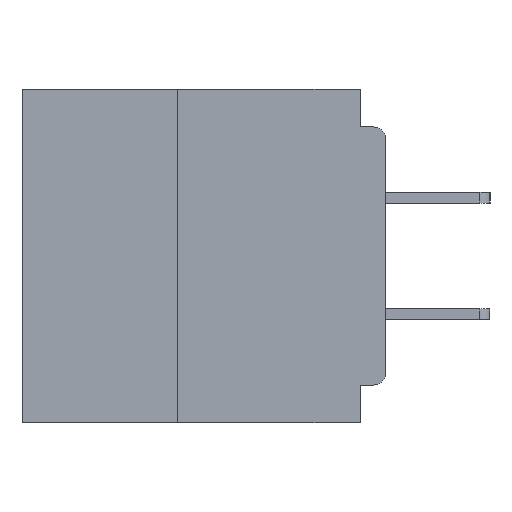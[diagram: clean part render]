
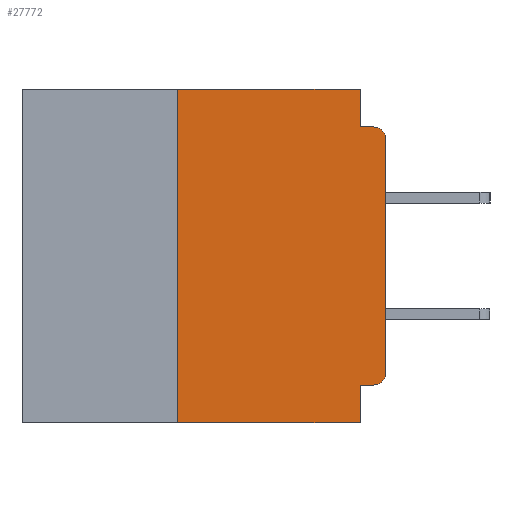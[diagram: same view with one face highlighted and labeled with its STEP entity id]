
A CAD part, left-side view. The second image highlights one B-rep face of the part: STEP entity #27772.
In plain terms, the highlighted planar face has unit normal (-1, 0, 0).
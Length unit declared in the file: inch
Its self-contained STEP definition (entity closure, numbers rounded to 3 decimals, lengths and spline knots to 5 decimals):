
#94 = VECTOR ( 'NONE', #56220, 39.37008 ) ;
#1191 = EDGE_CURVE ( 'NONE', #36905, #11573, #17959, .T. ) ;
#1698 = CARTESIAN_POINT ( 'NONE',  ( 0., 0.437, 0. ) ) ;
#2659 = VECTOR ( 'NONE', #55252, 39.37008 ) ;
#3322 = DIRECTION ( 'NONE',  ( 0., -1., 0. ) ) ;
#4088 = LINE ( 'NONE', #19762, #2659 ) ;
#4340 = CARTESIAN_POINT ( 'NONE',  ( 0., 0.015, -0.34 ) ) ;
#6059 = DIRECTION ( 'NONE',  ( 0., -1., 0. ) ) ;
#6978 = ORIENTED_EDGE ( 'NONE', *, *, #24669, .F. ) ;
#7606 = VERTEX_POINT ( 'NONE', #56738 ) ;
#8881 = VERTEX_POINT ( 'NONE', #48697 ) ;
#8902 = DIRECTION ( 'NONE',  ( 0., 0., -1. ) ) ;
#9409 = DIRECTION ( 'NONE',  ( 0., 0., -1. ) ) ;
#9584 = ORIENTED_EDGE ( 'NONE', *, *, #54353, .F. ) ;
#10184 = ORIENTED_EDGE ( 'NONE', *, *, #32303, .T. ) ;
#10202 = DIRECTION ( 'NONE',  ( -1., 0., 0. ) ) ;
#10310 = CARTESIAN_POINT ( 'NONE',  ( 0., 0., -0.34 ) ) ;
#10377 = CARTESIAN_POINT ( 'NONE',  ( 0., 0., 0. ) ) ;
#10418 = CARTESIAN_POINT ( 'NONE',  ( 0., 0.031, -0.045 ) ) ;
#10427 = CARTESIAN_POINT ( 'NONE',  ( 0., 0.015, -0.06 ) ) ;
#10504 = LINE ( 'NONE', #31536, #54953 ) ;
#10803 = PLANE ( 'NONE',  #57259 ) ;
#11276 = ORIENTED_EDGE ( 'NONE', *, *, #25697, .F. ) ;
#11492 = EDGE_CURVE ( 'NONE', #44159, #36905, #55331, .T. ) ;
#11573 = VERTEX_POINT ( 'NONE', #42089 ) ;
#12667 = ORIENTED_EDGE ( 'NONE', *, *, #37533, .F. ) ;
#14082 = CARTESIAN_POINT ( 'NONE',  ( 0., 0.031, -0.4 ) ) ;
#15101 = CARTESIAN_POINT ( 'NONE',  ( 0., 0.437, -0.4 ) ) ;
#15177 = EDGE_CURVE ( 'NONE', #23850, #37865, #10504, .T. ) ;
#15303 = DIRECTION ( 'NONE',  ( 1., 0., 0. ) ) ;
#15924 = AXIS2_PLACEMENT_3D ( 'NONE', #10427, #10202, #9409 ) ;
#16130 = ORIENTED_EDGE ( 'NONE', *, *, #48444, .T. ) ;
#17959 = CIRCLE ( 'NONE', #15924, 0.015 ) ;
#19640 = CARTESIAN_POINT ( 'NONE',  ( 0., 0.031, -0.4 ) ) ;
#19762 = CARTESIAN_POINT ( 'NONE',  ( 0., 0.437, 0. ) ) ;
#20561 = EDGE_CURVE ( 'NONE', #8881, #45886, #46834, .T. ) ;
#21543 = CARTESIAN_POINT ( 'NONE',  ( 0., 0.25, -0.4 ) ) ;
#21859 = ORIENTED_EDGE ( 'NONE', *, *, #1191, .T. ) ;
#23850 = VERTEX_POINT ( 'NONE', #44848 ) ;
#24336 = EDGE_LOOP ( 'NONE', ( #33076, #21859, #11276, #45212, #12667, #9584, #16130, #6978, #37281, #10184 ) ) ;
#24669 = EDGE_CURVE ( 'NONE', #37865, #31959, #56755, .T. ) ;
#25697 = EDGE_CURVE ( 'NONE', #45886, #11573, #53175, .T. ) ;
#27285 = DIRECTION ( 'NONE',  ( 0., 1., 0. ) ) ;
#27772 = ADVANCED_FACE ( 'NONE', ( #42570 ), #10803, .F. ) ;
#31536 = CARTESIAN_POINT ( 'NONE',  ( 0., 0., -0.355 ) ) ;
#31767 = VECTOR ( 'NONE', #50371, 39.37008 ) ;
#31959 = VERTEX_POINT ( 'NONE', #19640 ) ;
#32239 = VECTOR ( 'NONE', #51934, 39.37008 ) ;
#32303 = EDGE_CURVE ( 'NONE', #23850, #44159, #39560, .T. ) ;
#33076 = ORIENTED_EDGE ( 'NONE', *, *, #11492, .T. ) ;
#34413 = LINE ( 'NONE', #38454, #94 ) ;
#35580 = DIRECTION ( 'NONE',  ( -1., 0., 0. ) ) ;
#35781 = VERTEX_POINT ( 'NONE', #21543 ) ;
#36905 = VERTEX_POINT ( 'NONE', #55708 ) ;
#37281 = ORIENTED_EDGE ( 'NONE', *, *, #15177, .F. ) ;
#37533 = EDGE_CURVE ( 'NONE', #7606, #8881, #4088, .T. ) ;
#37865 = VERTEX_POINT ( 'NONE', #48659 ) ;
#38454 = CARTESIAN_POINT ( 'NONE',  ( 0., 0.25, -0.4 ) ) ;
#39560 = CIRCLE ( 'NONE', #56332, 0.015 ) ;
#40724 = DIRECTION ( 'NONE',  ( 0., 0., -1. ) ) ;
#41441 = VECTOR ( 'NONE', #3322, 39.37008 ) ;
#41519 = LINE ( 'NONE', #15101, #50481 ) ;
#42089 = CARTESIAN_POINT ( 'NONE',  ( 0., 0.015, -0.045 ) ) ;
#42570 = FACE_OUTER_BOUND ( 'NONE', #24336, .T. ) ;
#43653 = VECTOR ( 'NONE', #40724, 39.37008 ) ;
#44159 = VERTEX_POINT ( 'NONE', #10310 ) ;
#44848 = CARTESIAN_POINT ( 'NONE',  ( 0., 0.015, -0.355 ) ) ;
#45212 = ORIENTED_EDGE ( 'NONE', *, *, #20561, .F. ) ;
#45886 = VERTEX_POINT ( 'NONE', #10418 ) ;
#46395 = DIRECTION ( 'NONE',  ( 0., 0., -1. ) ) ;
#46834 = LINE ( 'NONE', #56564, #32239 ) ;
#47769 = CARTESIAN_POINT ( 'NONE',  ( 0., 0., -0.045 ) ) ;
#48444 = EDGE_CURVE ( 'NONE', #35781, #31959, #41519, .T. ) ;
#48659 = CARTESIAN_POINT ( 'NONE',  ( 0., 0.031, -0.355 ) ) ;
#48697 = CARTESIAN_POINT ( 'NONE',  ( 0., 0.031, 0. ) ) ;
#50371 = DIRECTION ( 'NONE',  ( 0., 0., 1. ) ) ;
#50481 = VECTOR ( 'NONE', #6059, 39.37008 ) ;
#51934 = DIRECTION ( 'NONE',  ( 0., 0., -1. ) ) ;
#53175 = LINE ( 'NONE', #47769, #41441 ) ;
#54353 = EDGE_CURVE ( 'NONE', #35781, #7606, #34413, .T. ) ;
#54953 = VECTOR ( 'NONE', #27285, 39.37008 ) ;
#55252 = DIRECTION ( 'NONE',  ( 0., -1., 0. ) ) ;
#55331 = LINE ( 'NONE', #10377, #31767 ) ;
#55708 = CARTESIAN_POINT ( 'NONE',  ( 0., 0., -0.06 ) ) ;
#56220 = DIRECTION ( 'NONE',  ( 0., 0., 1. ) ) ;
#56332 = AXIS2_PLACEMENT_3D ( 'NONE', #4340, #35580, #8902 ) ;
#56564 = CARTESIAN_POINT ( 'NONE',  ( 0., 0.031, 0. ) ) ;
#56738 = CARTESIAN_POINT ( 'NONE',  ( 0., 0.25, 0. ) ) ;
#56755 = LINE ( 'NONE', #14082, #43653 ) ;
#57259 = AXIS2_PLACEMENT_3D ( 'NONE', #1698, #15303, #46395 ) ;
